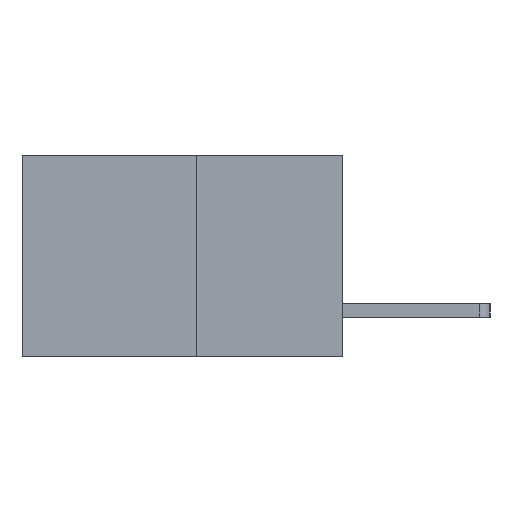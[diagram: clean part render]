
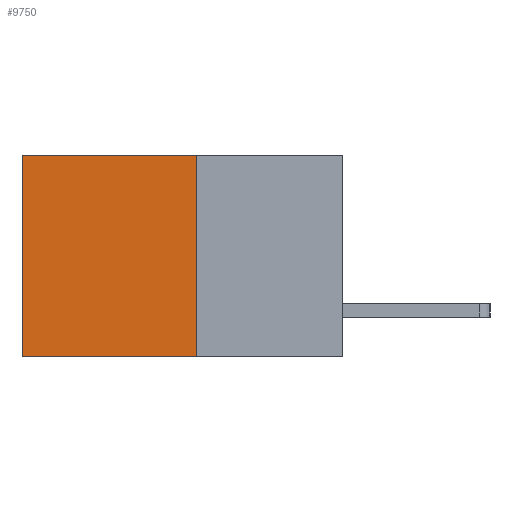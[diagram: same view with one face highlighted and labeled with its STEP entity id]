
A CAD part, left-side view. The second image highlights one B-rep face of the part: STEP entity #9750.
In plain terms, the highlighted planar face has unit normal (-1, 0, 0).
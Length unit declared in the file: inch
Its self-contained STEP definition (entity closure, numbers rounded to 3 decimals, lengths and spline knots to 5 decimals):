
#363 = LINE ( 'NONE', #7612, #4564 ) ;
#746 = AXIS2_PLACEMENT_3D ( 'NONE', #10518, #1873, #7984 ) ;
#1240 = FACE_OUTER_BOUND ( 'NONE', #6017, .T. ) ;
#1267 = VECTOR ( 'NONE', #2416, 39.37008 ) ;
#1651 = CARTESIAN_POINT ( 'NONE',  ( 0.277, 0.59, -0.37 ) ) ;
#1771 = VERTEX_POINT ( 'NONE', #8657 ) ;
#1873 = DIRECTION ( 'NONE',  ( 1., 0., 0. ) ) ;
#2416 = DIRECTION ( 'NONE',  ( 0., 0., -1. ) ) ;
#2914 = CARTESIAN_POINT ( 'NONE',  ( 0.277, 0.27, 0. ) ) ;
#3171 = EDGE_CURVE ( 'NONE', #4548, #1771, #7835, .T. ) ;
#3172 = CARTESIAN_POINT ( 'NONE',  ( 0.277, 0.27, -0.37 ) ) ;
#3303 = DIRECTION ( 'NONE',  ( 0., 1., 0. ) ) ;
#3625 = DIRECTION ( 'NONE',  ( 0., 0., -1. ) ) ;
#4129 = ORIENTED_EDGE ( 'NONE', *, *, #5428, .F. ) ;
#4548 = VERTEX_POINT ( 'NONE', #2914 ) ;
#4564 = VECTOR ( 'NONE', #3303, 39.37008 ) ;
#4873 = DIRECTION ( 'NONE',  ( 0., 1., 0. ) ) ;
#5428 = EDGE_CURVE ( 'NONE', #1771, #7296, #363, .T. ) ;
#5734 = CARTESIAN_POINT ( 'NONE',  ( 0.277, 0.27, 0. ) ) ;
#5979 = LINE ( 'NONE', #6752, #1267 ) ;
#6017 = EDGE_LOOP ( 'NONE', ( #7171, #4129, #6166, #9892 ) ) ;
#6166 = ORIENTED_EDGE ( 'NONE', *, *, #3171, .F. ) ;
#6570 = EDGE_CURVE ( 'NONE', #4548, #8800, #8661, .T. ) ;
#6711 = CARTESIAN_POINT ( 'NONE',  ( 0.277, 0.59, 0. ) ) ;
#6752 = CARTESIAN_POINT ( 'NONE',  ( 0.277, 0.59, -0.37 ) ) ;
#7095 = PLANE ( 'NONE',  #746 ) ;
#7171 = ORIENTED_EDGE ( 'NONE', *, *, #8829, .T. ) ;
#7296 = VERTEX_POINT ( 'NONE', #1651 ) ;
#7553 = VECTOR ( 'NONE', #3625, 39.37008 ) ;
#7612 = CARTESIAN_POINT ( 'NONE',  ( 0.277, 0.27, -0.37 ) ) ;
#7835 = LINE ( 'NONE', #3172, #7553 ) ;
#7984 = DIRECTION ( 'NONE',  ( 0., 0., -1. ) ) ;
#8657 = CARTESIAN_POINT ( 'NONE',  ( 0.277, 0.27, -0.37 ) ) ;
#8661 = LINE ( 'NONE', #5734, #10678 ) ;
#8800 = VERTEX_POINT ( 'NONE', #6711 ) ;
#8829 = EDGE_CURVE ( 'NONE', #8800, #7296, #5979, .T. ) ;
#9750 = ADVANCED_FACE ( 'NONE', ( #1240 ), #7095, .F. ) ;
#9892 = ORIENTED_EDGE ( 'NONE', *, *, #6570, .T. ) ;
#10518 = CARTESIAN_POINT ( 'NONE',  ( 0.277, 0.27, -0.37 ) ) ;
#10678 = VECTOR ( 'NONE', #4873, 39.37008 ) ;
